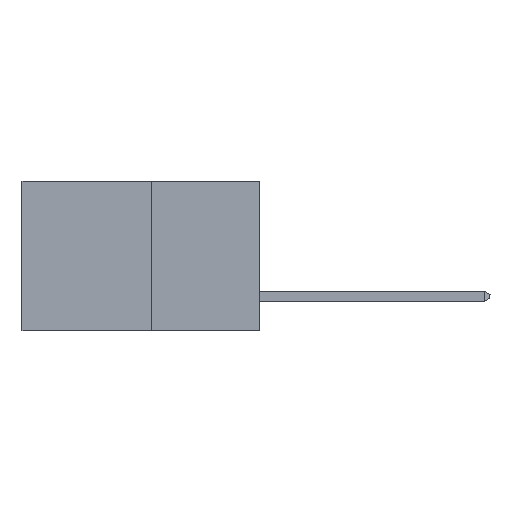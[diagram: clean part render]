
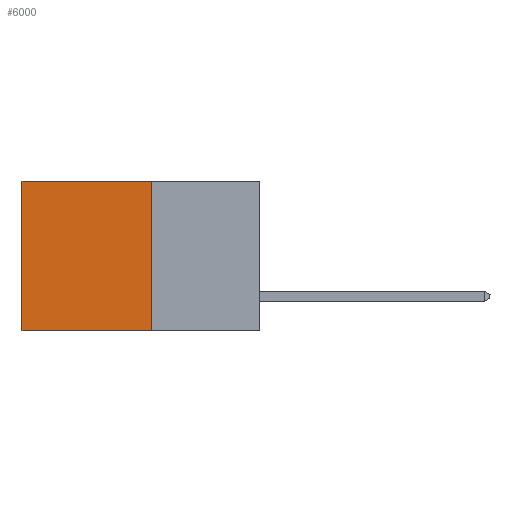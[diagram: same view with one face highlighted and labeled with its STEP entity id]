
A CAD part, left-side view. The second image highlights one B-rep face of the part: STEP entity #6000.
In plain terms, the highlighted planar face has unit normal (-1, 0, 0).
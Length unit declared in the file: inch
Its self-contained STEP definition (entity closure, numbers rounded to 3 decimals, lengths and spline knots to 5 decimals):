
#14 = ORIENTED_EDGE ( 'NONE', *, *, #4076, .F. ) ;
#718 = CARTESIAN_POINT ( 'NONE',  ( 0.277, 0.27, 0. ) ) ;
#1337 = VECTOR ( 'NONE', #3813, 39.37008 ) ;
#1663 = DIRECTION ( 'NONE',  ( 1., 0., 0. ) ) ;
#1674 = DIRECTION ( 'NONE',  ( 0., 0., -1. ) ) ;
#1852 = PLANE ( 'NONE',  #10705 ) ;
#1900 = CARTESIAN_POINT ( 'NONE',  ( 0.277, 0.27, -0.37 ) ) ;
#1908 = ORIENTED_EDGE ( 'NONE', *, *, #4972, .T. ) ;
#2293 = VERTEX_POINT ( 'NONE', #8985 ) ;
#2801 = DIRECTION ( 'NONE',  ( 0., 1., 0. ) ) ;
#2900 = CARTESIAN_POINT ( 'NONE',  ( 0.277, 0.27, -0.37 ) ) ;
#2979 = VERTEX_POINT ( 'NONE', #4253 ) ;
#3119 = EDGE_CURVE ( 'NONE', #2979, #10190, #6655, .T. ) ;
#3146 = DIRECTION ( 'NONE',  ( 0., 0., -1. ) ) ;
#3197 = CARTESIAN_POINT ( 'NONE',  ( 0.277, 0.27, -0.37 ) ) ;
#3813 = DIRECTION ( 'NONE',  ( 0., 0., -1. ) ) ;
#4076 = EDGE_CURVE ( 'NONE', #2293, #2979, #6513, .T. ) ;
#4230 = VECTOR ( 'NONE', #2801, 39.37008 ) ;
#4253 = CARTESIAN_POINT ( 'NONE',  ( 0.277, 0.27, -0.37 ) ) ;
#4764 = CARTESIAN_POINT ( 'NONE',  ( 0.277, 0.59, -0.37 ) ) ;
#4972 = EDGE_CURVE ( 'NONE', #8013, #10190, #8063, .T. ) ;
#5937 = LINE ( 'NONE', #718, #8653 ) ;
#6000 = ADVANCED_FACE ( 'NONE', ( #11067 ), #1852, .F. ) ;
#6437 = CARTESIAN_POINT ( 'NONE',  ( 0.277, 0.59, 0. ) ) ;
#6513 = LINE ( 'NONE', #3197, #10983 ) ;
#6567 = ORIENTED_EDGE ( 'NONE', *, *, #9429, .T. ) ;
#6655 = LINE ( 'NONE', #2900, #4230 ) ;
#7090 = DIRECTION ( 'NONE',  ( 0., 1., 0. ) ) ;
#7350 = ORIENTED_EDGE ( 'NONE', *, *, #3119, .F. ) ;
#7716 = EDGE_LOOP ( 'NONE', ( #1908, #7350, #14, #6567 ) ) ;
#8013 = VERTEX_POINT ( 'NONE', #6437 ) ;
#8063 = LINE ( 'NONE', #4764, #1337 ) ;
#8653 = VECTOR ( 'NONE', #7090, 39.37008 ) ;
#8985 = CARTESIAN_POINT ( 'NONE',  ( 0.277, 0.27, 0. ) ) ;
#9429 = EDGE_CURVE ( 'NONE', #2293, #8013, #5937, .T. ) ;
#9944 = CARTESIAN_POINT ( 'NONE',  ( 0.277, 0.59, -0.37 ) ) ;
#10190 = VERTEX_POINT ( 'NONE', #9944 ) ;
#10705 = AXIS2_PLACEMENT_3D ( 'NONE', #1900, #1663, #1674 ) ;
#10983 = VECTOR ( 'NONE', #3146, 39.37008 ) ;
#11067 = FACE_OUTER_BOUND ( 'NONE', #7716, .T. ) ;
